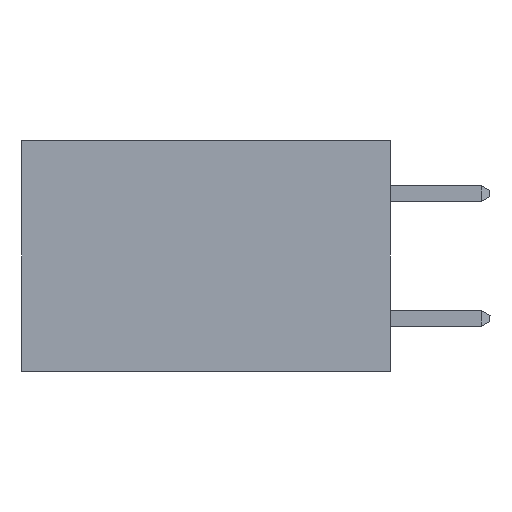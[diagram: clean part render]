
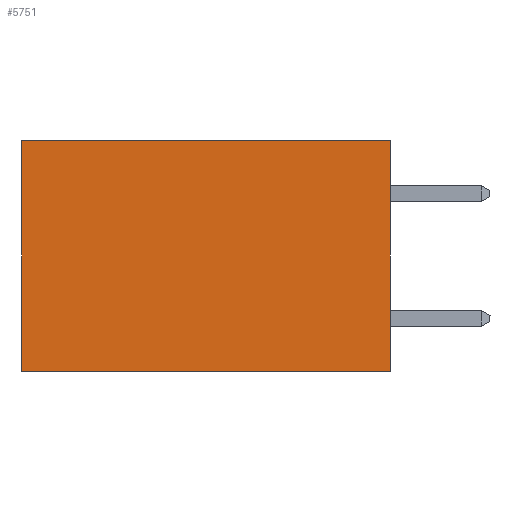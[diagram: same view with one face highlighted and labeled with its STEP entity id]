
A CAD part, left-side view. The second image highlights one B-rep face of the part: STEP entity #5751.
In plain terms, the highlighted planar face has unit normal (-1, 0, 0).
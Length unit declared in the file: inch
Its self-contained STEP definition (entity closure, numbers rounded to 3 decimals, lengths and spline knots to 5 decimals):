
#7 = CARTESIAN_POINT ( 'NONE',  ( 0.277, 0., -0.37 ) ) ;
#271 = LINE ( 'NONE', #328, #2555 ) ;
#328 = CARTESIAN_POINT ( 'NONE',  ( 0.277, 0.59, -0.37 ) ) ;
#373 = EDGE_CURVE ( 'NONE', #9977, #5854, #6300, .T. ) ;
#545 = EDGE_CURVE ( 'NONE', #5854, #5290, #271, .T. ) ;
#766 = DIRECTION ( 'NONE',  ( 0., 0., -1. ) ) ;
#773 = AXIS2_PLACEMENT_3D ( 'NONE', #2633, #6115, #766 ) ;
#1338 = CARTESIAN_POINT ( 'NONE',  ( 0.277, 0.59, -0.37 ) ) ;
#2005 = ORIENTED_EDGE ( 'NONE', *, *, #2842, .F. ) ;
#2166 = EDGE_LOOP ( 'NONE', ( #6224, #2005, #2310, #6499 ) ) ;
#2310 = ORIENTED_EDGE ( 'NONE', *, *, #2864, .F. ) ;
#2555 = VECTOR ( 'NONE', #4863, 39.37008 ) ;
#2633 = CARTESIAN_POINT ( 'NONE',  ( 0.277, 0., -0.37 ) ) ;
#2842 = EDGE_CURVE ( 'NONE', #8607, #5290, #7397, .T. ) ;
#2864 = EDGE_CURVE ( 'NONE', #9977, #8607, #6977, .T. ) ;
#4863 = DIRECTION ( 'NONE',  ( 0., 0., -1. ) ) ;
#5290 = VERTEX_POINT ( 'NONE', #1338 ) ;
#5313 = PLANE ( 'NONE',  #773 ) ;
#5751 = ADVANCED_FACE ( 'NONE', ( #9529 ), #5313, .F. ) ;
#5854 = VERTEX_POINT ( 'NONE', #7595 ) ;
#6115 = DIRECTION ( 'NONE',  ( 1., 0., 0. ) ) ;
#6224 = ORIENTED_EDGE ( 'NONE', *, *, #545, .T. ) ;
#6300 = LINE ( 'NONE', #8608, #7887 ) ;
#6499 = ORIENTED_EDGE ( 'NONE', *, *, #373, .T. ) ;
#6977 = LINE ( 'NONE', #7755, #10072 ) ;
#7193 = VECTOR ( 'NONE', #8063, 39.37008 ) ;
#7397 = LINE ( 'NONE', #8091, #7193 ) ;
#7400 = CARTESIAN_POINT ( 'NONE',  ( 0.277, 0., 0. ) ) ;
#7595 = CARTESIAN_POINT ( 'NONE',  ( 0.277, 0.59, 0. ) ) ;
#7733 = DIRECTION ( 'NONE',  ( 0., 0., -1. ) ) ;
#7755 = CARTESIAN_POINT ( 'NONE',  ( 0.277, 0., -0.37 ) ) ;
#7887 = VECTOR ( 'NONE', #8923, 39.37008 ) ;
#8063 = DIRECTION ( 'NONE',  ( 0., 1., 0. ) ) ;
#8091 = CARTESIAN_POINT ( 'NONE',  ( 0.277, 0., -0.37 ) ) ;
#8607 = VERTEX_POINT ( 'NONE', #7 ) ;
#8608 = CARTESIAN_POINT ( 'NONE',  ( 0.277, 0., 0. ) ) ;
#8923 = DIRECTION ( 'NONE',  ( 0., 1., 0. ) ) ;
#9529 = FACE_OUTER_BOUND ( 'NONE', #2166, .T. ) ;
#9977 = VERTEX_POINT ( 'NONE', #7400 ) ;
#10072 = VECTOR ( 'NONE', #7733, 39.37008 ) ;
